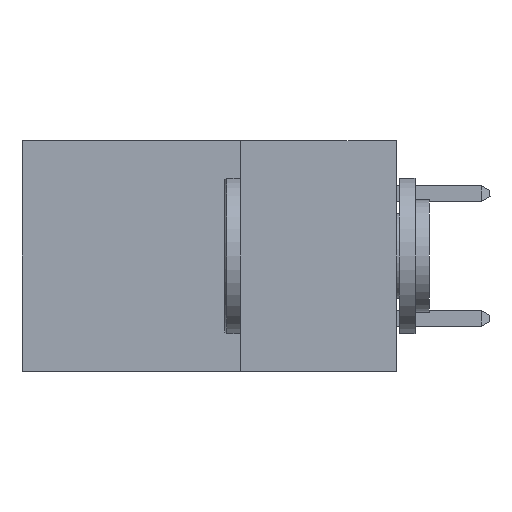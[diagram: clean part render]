
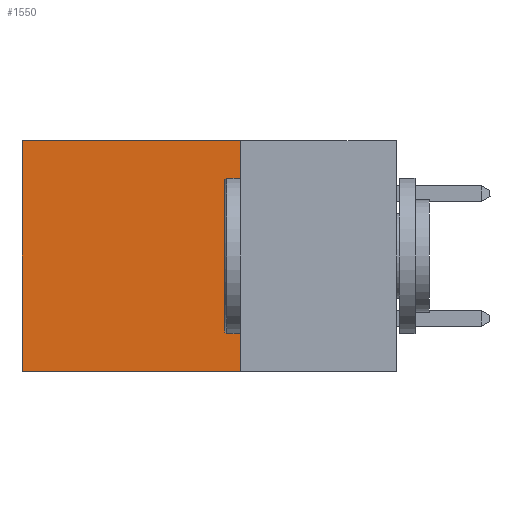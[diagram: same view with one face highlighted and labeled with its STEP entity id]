
A CAD part, left-side view. The second image highlights one B-rep face of the part: STEP entity #1550.
In plain terms, the highlighted planar face has unit normal (-1, 0, 0).
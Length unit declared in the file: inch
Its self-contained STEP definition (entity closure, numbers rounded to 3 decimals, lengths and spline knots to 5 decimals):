
#1483 = EDGE_CURVE ( 'NONE', #17898, #3714, #15260, .T. ) ;
#1550 = ADVANCED_FACE ( 'NONE', ( #6885 ), #11941, .F. ) ;
#1598 = DIRECTION ( 'NONE',  ( 0., 0., -1. ) ) ;
#3708 = CARTESIAN_POINT ( 'NONE',  ( 0.298, 0.25, 0. ) ) ;
#3714 = VERTEX_POINT ( 'NONE', #15779 ) ;
#4306 = EDGE_CURVE ( 'NONE', #17898, #15089, #20236, .T. ) ;
#4725 = ORIENTED_EDGE ( 'NONE', *, *, #4306, .F. ) ;
#6045 = LINE ( 'NONE', #15970, #15001 ) ;
#6170 = CARTESIAN_POINT ( 'NONE',  ( 0.298, 0.25, 0. ) ) ;
#6324 = EDGE_LOOP ( 'NONE', ( #22059, #9741, #4725, #20714 ) ) ;
#6885 = FACE_OUTER_BOUND ( 'NONE', #6324, .T. ) ;
#8120 = CARTESIAN_POINT ( 'NONE',  ( 0.298, 0.6, -0.37 ) ) ;
#8282 = AXIS2_PLACEMENT_3D ( 'NONE', #13518, #14102, #12400 ) ;
#9741 = ORIENTED_EDGE ( 'NONE', *, *, #16103, .F. ) ;
#10535 = VECTOR ( 'NONE', #14866, 39.37008 ) ;
#11697 = DIRECTION ( 'NONE',  ( 0., 0., -1. ) ) ;
#11811 = VECTOR ( 'NONE', #11697, 39.37008 ) ;
#11941 = PLANE ( 'NONE',  #8282 ) ;
#12400 = DIRECTION ( 'NONE',  ( 0., 0., -1. ) ) ;
#12502 = EDGE_CURVE ( 'NONE', #3714, #19162, #15959, .T. ) ;
#13450 = CARTESIAN_POINT ( 'NONE',  ( 0.298, 0.25, -0.37 ) ) ;
#13518 = CARTESIAN_POINT ( 'NONE',  ( 0.298, 0.25, 0. ) ) ;
#14102 = DIRECTION ( 'NONE',  ( 1., 0., 0. ) ) ;
#14866 = DIRECTION ( 'NONE',  ( 0., 1., 0. ) ) ;
#15001 = VECTOR ( 'NONE', #17706, 39.37008 ) ;
#15089 = VERTEX_POINT ( 'NONE', #13450 ) ;
#15260 = LINE ( 'NONE', #6170, #10535 ) ;
#15635 = VECTOR ( 'NONE', #1598, 39.37008 ) ;
#15779 = CARTESIAN_POINT ( 'NONE',  ( 0.298, 0.6, 0. ) ) ;
#15959 = LINE ( 'NONE', #22124, #11811 ) ;
#15970 = CARTESIAN_POINT ( 'NONE',  ( 0.298, 0.25, -0.37 ) ) ;
#16103 = EDGE_CURVE ( 'NONE', #15089, #19162, #6045, .T. ) ;
#17192 = CARTESIAN_POINT ( 'NONE',  ( 0.298, 0.25, 0. ) ) ;
#17706 = DIRECTION ( 'NONE',  ( 0., 1., 0. ) ) ;
#17898 = VERTEX_POINT ( 'NONE', #17192 ) ;
#19162 = VERTEX_POINT ( 'NONE', #8120 ) ;
#20236 = LINE ( 'NONE', #3708, #15635 ) ;
#20714 = ORIENTED_EDGE ( 'NONE', *, *, #1483, .T. ) ;
#22059 = ORIENTED_EDGE ( 'NONE', *, *, #12502, .T. ) ;
#22124 = CARTESIAN_POINT ( 'NONE',  ( 0.298, 0.6, 0. ) ) ;
